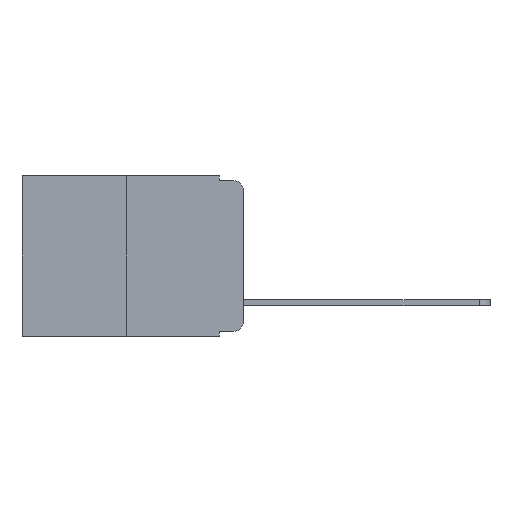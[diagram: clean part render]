
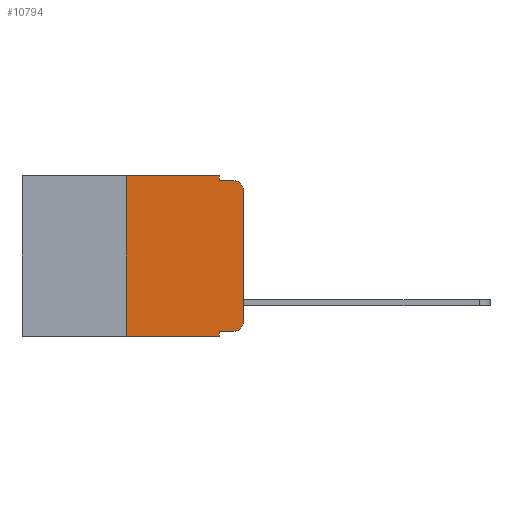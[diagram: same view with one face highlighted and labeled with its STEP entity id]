
A CAD part, left-side view. The second image highlights one B-rep face of the part: STEP entity #10794.
In plain terms, the highlighted planar face has unit normal (-1, 0, 0).
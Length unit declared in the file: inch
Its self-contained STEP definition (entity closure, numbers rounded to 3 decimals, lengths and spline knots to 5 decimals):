
#525 = EDGE_CURVE ( 'NONE', #14523, #12199, #11745, .T. ) ;
#672 = LINE ( 'NONE', #1285, #6665 ) ;
#673 = CARTESIAN_POINT ( 'NONE',  ( 0., 0.473, 0. ) ) ;
#775 = VERTEX_POINT ( 'NONE', #5978 ) ;
#817 = AXIS2_PLACEMENT_3D ( 'NONE', #673, #3448, #11428 ) ;
#828 = ORIENTED_EDGE ( 'NONE', *, *, #3834, .T. ) ;
#896 = VERTEX_POINT ( 'NONE', #2694 ) ;
#1083 = VERTEX_POINT ( 'NONE', #10868 ) ;
#1103 = CARTESIAN_POINT ( 'NONE',  ( 0., 0.02, -0.313 ) ) ;
#1285 = CARTESIAN_POINT ( 'NONE',  ( 0., 0.473, 0. ) ) ;
#1384 = EDGE_CURVE ( 'NONE', #1083, #775, #13693, .T. ) ;
#1462 = CARTESIAN_POINT ( 'NONE',  ( 0., 0., 0. ) ) ;
#1483 = VERTEX_POINT ( 'NONE', #4179 ) ;
#1700 = CARTESIAN_POINT ( 'NONE',  ( 0., 0.25, 0. ) ) ;
#1704 = DIRECTION ( 'NONE',  ( 0., 0., -1. ) ) ;
#1765 = DIRECTION ( 'NONE',  ( 0., 0., -1. ) ) ;
#1939 = FACE_OUTER_BOUND ( 'NONE', #8766, .T. ) ;
#2200 = EDGE_CURVE ( 'NONE', #775, #9531, #7026, .T. ) ;
#2346 = DIRECTION ( 'NONE',  ( 0., 0., -1. ) ) ;
#2393 = ORIENTED_EDGE ( 'NONE', *, *, #13975, .F. ) ;
#2694 = CARTESIAN_POINT ( 'NONE',  ( 0., 0., -0.313 ) ) ;
#2777 = ORIENTED_EDGE ( 'NONE', *, *, #12460, .T. ) ;
#2867 = CARTESIAN_POINT ( 'NONE',  ( 0., 0.051, 0. ) ) ;
#3032 = EDGE_CURVE ( 'NONE', #8451, #9531, #8110, .T. ) ;
#3448 = DIRECTION ( 'NONE',  ( 1., 0., 0. ) ) ;
#3473 = CARTESIAN_POINT ( 'NONE',  ( 0., 0.051, -0.01 ) ) ;
#3684 = VERTEX_POINT ( 'NONE', #8368 ) ;
#3710 = CARTESIAN_POINT ( 'NONE',  ( 0., 0.051, -0.333 ) ) ;
#3813 = DIRECTION ( 'NONE',  ( 0., -1., 0. ) ) ;
#3833 = DIRECTION ( 'NONE',  ( 0., -1., 0. ) ) ;
#3834 = EDGE_CURVE ( 'NONE', #896, #8451, #13608, .T. ) ;
#4179 = CARTESIAN_POINT ( 'NONE',  ( 0., 0.051, -0.343 ) ) ;
#4579 = CARTESIAN_POINT ( 'NONE',  ( 0., 0.25, 0. ) ) ;
#4686 = AXIS2_PLACEMENT_3D ( 'NONE', #10878, #10881, #1704 ) ;
#4806 = ORIENTED_EDGE ( 'NONE', *, *, #6695, .F. ) ;
#4914 = DIRECTION ( 'NONE',  ( 0., -1., 0. ) ) ;
#4916 = LINE ( 'NONE', #3710, #10682 ) ;
#5239 = VECTOR ( 'NONE', #1765, 39.37008 ) ;
#5296 = DIRECTION ( 'NONE',  ( 0., 0., 1. ) ) ;
#5503 = LINE ( 'NONE', #12880, #11212 ) ;
#5647 = CARTESIAN_POINT ( 'NONE',  ( 0., 0.02, -0.01 ) ) ;
#5978 = CARTESIAN_POINT ( 'NONE',  ( 0., 0.051, -0.01 ) ) ;
#6267 = VECTOR ( 'NONE', #3813, 39.37008 ) ;
#6340 = CARTESIAN_POINT ( 'NONE',  ( 0., 0.02, -0.333 ) ) ;
#6665 = VECTOR ( 'NONE', #4914, 39.37008 ) ;
#6695 = EDGE_CURVE ( 'NONE', #12199, #1083, #672, .T. ) ;
#7026 = LINE ( 'NONE', #3473, #6267 ) ;
#7307 = VERTEX_POINT ( 'NONE', #6340 ) ;
#7546 = ORIENTED_EDGE ( 'NONE', *, *, #2200, .F. ) ;
#8094 = PLANE ( 'NONE',  #817 ) ;
#8110 = CIRCLE ( 'NONE', #4686, 0.02 ) ;
#8358 = LINE ( 'NONE', #9993, #5239 ) ;
#8368 = CARTESIAN_POINT ( 'NONE',  ( 0., 0.051, -0.333 ) ) ;
#8451 = VERTEX_POINT ( 'NONE', #11814 ) ;
#8524 = DIRECTION ( 'NONE',  ( 0., 0., -1. ) ) ;
#8766 = EDGE_LOOP ( 'NONE', ( #828, #13089, #7546, #13461, #4806, #13812, #11236, #2393, #11562, #2777 ) ) ;
#8848 = VECTOR ( 'NONE', #5296, 39.37008 ) ;
#9371 = DIRECTION ( 'NONE',  ( -1., 0., 0. ) ) ;
#9531 = VERTEX_POINT ( 'NONE', #5647 ) ;
#9824 = EDGE_CURVE ( 'NONE', #14523, #1483, #5503, .T. ) ;
#9993 = CARTESIAN_POINT ( 'NONE',  ( 0., 0.051, 0. ) ) ;
#10682 = VECTOR ( 'NONE', #12715, 39.37008 ) ;
#10726 = VECTOR ( 'NONE', #12549, 39.37008 ) ;
#10794 = ADVANCED_FACE ( 'NONE', ( #1939 ), #8094, .F. ) ;
#10868 = CARTESIAN_POINT ( 'NONE',  ( 0., 0.051, 0. ) ) ;
#10878 = CARTESIAN_POINT ( 'NONE',  ( 0., 0.02, -0.03 ) ) ;
#10881 = DIRECTION ( 'NONE',  ( -1., 0., 0. ) ) ;
#10956 = CARTESIAN_POINT ( 'NONE',  ( 0., 0.25, -0.343 ) ) ;
#11212 = VECTOR ( 'NONE', #3833, 39.37008 ) ;
#11236 = ORIENTED_EDGE ( 'NONE', *, *, #9824, .T. ) ;
#11428 = DIRECTION ( 'NONE',  ( 0., 0., -1. ) ) ;
#11562 = ORIENTED_EDGE ( 'NONE', *, *, #13211, .T. ) ;
#11745 = LINE ( 'NONE', #4579, #8848 ) ;
#11814 = CARTESIAN_POINT ( 'NONE',  ( 0., 0., -0.03 ) ) ;
#12199 = VERTEX_POINT ( 'NONE', #1700 ) ;
#12460 = EDGE_CURVE ( 'NONE', #7307, #896, #14045, .T. ) ;
#12549 = DIRECTION ( 'NONE',  ( 0., 0., 1. ) ) ;
#12715 = DIRECTION ( 'NONE',  ( 0., -1., 0. ) ) ;
#12880 = CARTESIAN_POINT ( 'NONE',  ( 0., 0.473, -0.343 ) ) ;
#13089 = ORIENTED_EDGE ( 'NONE', *, *, #3032, .T. ) ;
#13211 = EDGE_CURVE ( 'NONE', #3684, #7307, #4916, .T. ) ;
#13461 = ORIENTED_EDGE ( 'NONE', *, *, #1384, .F. ) ;
#13608 = LINE ( 'NONE', #1462, #10726 ) ;
#13693 = LINE ( 'NONE', #2867, #14373 ) ;
#13812 = ORIENTED_EDGE ( 'NONE', *, *, #525, .F. ) ;
#13975 = EDGE_CURVE ( 'NONE', #3684, #1483, #8358, .T. ) ;
#14045 = CIRCLE ( 'NONE', #14487, 0.02 ) ;
#14373 = VECTOR ( 'NONE', #8524, 39.37008 ) ;
#14487 = AXIS2_PLACEMENT_3D ( 'NONE', #1103, #9371, #2346 ) ;
#14523 = VERTEX_POINT ( 'NONE', #10956 ) ;
